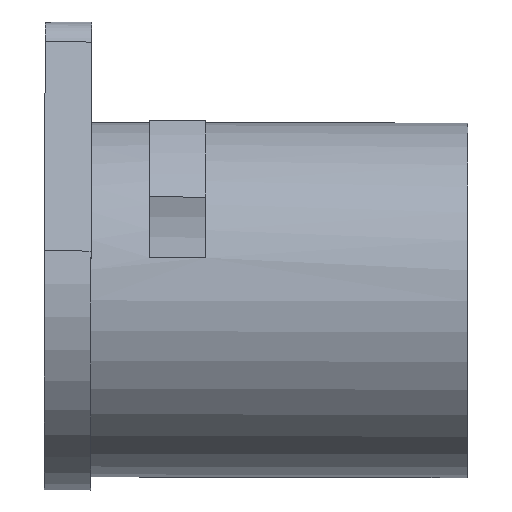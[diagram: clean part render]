
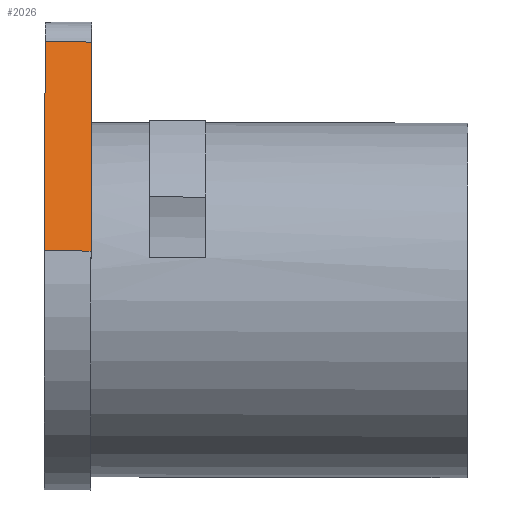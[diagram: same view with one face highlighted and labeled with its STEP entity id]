
A CAD part, left-side view. The second image highlights one B-rep face of the part: STEP entity #2026.
In plain terms, the highlighted planar face has unit normal (-0.967, 0, 0.255).
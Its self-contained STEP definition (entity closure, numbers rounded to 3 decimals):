
#821 = PLANE('',#822);
#822 = AXIS2_PLACEMENT_3D('',#823,#824,#825);
#823 = CARTESIAN_POINT('',(-0.01,-2.316,
    2.141));
#824 = DIRECTION('',(0.,1.,
    0.002));
#825 = DIRECTION('',(1.,0.,
    0.004));
#1085 = VERTEX_POINT('',#1086);
#1086 = CARTESIAN_POINT('',(-9.212,-2.313,
    2.419));
#1105 = CYLINDRICAL_SURFACE('',#1106,9.525);
#1106 = AXIS2_PLACEMENT_3D('',#1107,#1108,#1109);
#1107 = CARTESIAN_POINT('',(0.,0.,0.));
#1108 = DIRECTION('',(0.,-1.,
    -0.002));
#1109 = DIRECTION('',(0.004,0.002,
    -1.));
#1139 = EDGE_CURVE('',#1140,#1085,#1142,.T.);
#1140 = VERTEX_POINT('',#1141);
#1141 = CARTESIAN_POINT('',(-6.469,-2.336,
    12.841));
#1142 = SURFACE_CURVE('',#1143,(#1147,#1154),.PCURVE_S1.);
#1143 = LINE('',#1144,#1145);
#1144 = CARTESIAN_POINT('',(-9.212,-2.313,
    2.419));
#1145 = VECTOR('',#1146,1.);
#1146 = DIRECTION('',(-0.255,0.002,
    -0.967));
#1147 = PCURVE('',#821,#1148);
#1148 = DEFINITIONAL_REPRESENTATION('',(#1149),#1153);
#1149 = LINE('',#1150,#1151);
#1150 = CARTESIAN_POINT('',(-9.2,-0.32));
#1151 = VECTOR('',#1152,1.);
#1152 = DIRECTION('',(-0.259,0.966));
#1153 = ( GEOMETRIC_REPRESENTATION_CONTEXT(2) 
PARAMETRIC_REPRESENTATION_CONTEXT() REPRESENTATION_CONTEXT('2D SPACE',''
  ) );
#1154 = PCURVE('',#1155,#1160);
#1155 = PLANE('',#1156);
#1156 = AXIS2_PLACEMENT_3D('',#1157,#1158,#1159);
#1157 = CARTESIAN_POINT('',(-6.469,-0.025,
    12.846));
#1158 = DIRECTION('',(-0.967,0.,
    0.255));
#1159 = DIRECTION('',(-0.255,0.002,-0.967
    ));
#1160 = DEFINITIONAL_REPRESENTATION('',(#1161),#1165);
#1161 = LINE('',#1162,#1163);
#1162 = CARTESIAN_POINT('',(10.777,2.311));
#1163 = VECTOR('',#1164,1.);
#1164 = DIRECTION('',(1.,0.));
#1165 = ( GEOMETRIC_REPRESENTATION_CONTEXT(2) 
PARAMETRIC_REPRESENTATION_CONTEXT() REPRESENTATION_CONTEXT('2D SPACE',''
  ) );
#1188 = CYLINDRICAL_SURFACE('',#1189,1.27);
#1189 = AXIS2_PLACEMENT_3D('',#1190,#1191,#1192);
#1190 = CARTESIAN_POINT('',(-5.24,-0.024,
    12.523));
#1191 = DIRECTION('',(0.,-1.,
    -0.002));
#1192 = DIRECTION('',(-0.967,0.,
    0.255));
#1531 = PLANE('',#1532);
#1532 = AXIS2_PLACEMENT_3D('',#1533,#1534,#1535);
#1533 = CARTESIAN_POINT('',(-0.01,-0.004,
    2.146));
#1534 = DIRECTION('',(0.,1.,
    0.002));
#1535 = DIRECTION('',(1.,0.,
    0.004));
#1843 = VERTEX_POINT('',#1844);
#1844 = CARTESIAN_POINT('',(-9.211,-0.002,
    2.424));
#1890 = EDGE_CURVE('',#1843,#1085,#1891,.T.);
#1891 = SURFACE_CURVE('',#1892,(#1896,#1925),.PCURVE_S1.);
#1892 = LINE('',#1893,#1894);
#1893 = CARTESIAN_POINT('',(-9.211,-0.002,
    2.424));
#1894 = VECTOR('',#1895,1.);
#1895 = DIRECTION('',(0.,-1.,
    -0.002));
#1896 = PCURVE('',#1105,#1897);
#1897 = DEFINITIONAL_REPRESENTATION('',(#1898),#1924);
#1898 = B_SPLINE_CURVE_WITH_KNOTS('',3,(#1899,#1900,#1901,#1902,#1903,
    #1904,#1905,#1906,#1907,#1908,#1909,#1910,#1911,#1912,#1913,#1914,
    #1915,#1916,#1917,#1918,#1919,#1920,#1921,#1922,#1923),
  .UNSPECIFIED.,.F.,.F.,(4,1,1,1,1,1,1,1,1,1,1,1,1,1,1,1,1,1,1,1,1,1,4),
  (0.,0.105,0.21,0.315,0.42,
    0.525,0.63,0.735,0.841,
    0.946,1.051,1.156,1.261,1.366,
    1.471,1.576,1.681,1.786,
    1.891,1.996,2.101,2.206,2.311),
  .UNSPECIFIED.);
#1899 = CARTESIAN_POINT('',(-1.833,0.));
#1900 = CARTESIAN_POINT('',(-1.833,0.035));
#1901 = CARTESIAN_POINT('',(-1.833,0.105));
#1902 = CARTESIAN_POINT('',(-1.833,0.21));
#1903 = CARTESIAN_POINT('',(-1.833,0.315));
#1904 = CARTESIAN_POINT('',(-1.833,0.42));
#1905 = CARTESIAN_POINT('',(-1.833,0.525));
#1906 = CARTESIAN_POINT('',(-1.833,0.63));
#1907 = CARTESIAN_POINT('',(-1.833,0.735));
#1908 = CARTESIAN_POINT('',(-1.833,0.841));
#1909 = CARTESIAN_POINT('',(-1.833,0.946));
#1910 = CARTESIAN_POINT('',(-1.833,1.051));
#1911 = CARTESIAN_POINT('',(-1.833,1.156));
#1912 = CARTESIAN_POINT('',(-1.833,1.261));
#1913 = CARTESIAN_POINT('',(-1.833,1.366));
#1914 = CARTESIAN_POINT('',(-1.833,1.471));
#1915 = CARTESIAN_POINT('',(-1.833,1.576));
#1916 = CARTESIAN_POINT('',(-1.833,1.681));
#1917 = CARTESIAN_POINT('',(-1.833,1.786));
#1918 = CARTESIAN_POINT('',(-1.833,1.891));
#1919 = CARTESIAN_POINT('',(-1.833,1.996));
#1920 = CARTESIAN_POINT('',(-1.833,2.101));
#1921 = CARTESIAN_POINT('',(-1.833,2.206));
#1922 = CARTESIAN_POINT('',(-1.833,2.276));
#1923 = CARTESIAN_POINT('',(-1.833,2.311));
#1924 = ( GEOMETRIC_REPRESENTATION_CONTEXT(2) 
PARAMETRIC_REPRESENTATION_CONTEXT() REPRESENTATION_CONTEXT('2D SPACE',''
  ) );
#1925 = PCURVE('',#1155,#1926);
#1926 = DEFINITIONAL_REPRESENTATION('',(#1927),#1931);
#1927 = LINE('',#1928,#1929);
#1928 = CARTESIAN_POINT('',(10.777,0.));
#1929 = VECTOR('',#1930,1.);
#1930 = DIRECTION('',(0.,1.));
#1931 = ( GEOMETRIC_REPRESENTATION_CONTEXT(2) 
PARAMETRIC_REPRESENTATION_CONTEXT() REPRESENTATION_CONTEXT('2D SPACE',''
  ) );
#1937 = VERTEX_POINT('',#1938);
#1938 = CARTESIAN_POINT('',(-6.469,-0.025,
    12.846));
#1982 = EDGE_CURVE('',#1937,#1140,#1983,.T.);
#1983 = SURFACE_CURVE('',#1984,(#1988,#2017),.PCURVE_S1.);
#1984 = LINE('',#1985,#1986);
#1985 = CARTESIAN_POINT('',(-6.469,-0.025,
    12.846));
#1986 = VECTOR('',#1987,1.);
#1987 = DIRECTION('',(0.,-1.,
    -0.002));
#1988 = PCURVE('',#1188,#1989);
#1989 = DEFINITIONAL_REPRESENTATION('',(#1990),#2016);
#1990 = B_SPLINE_CURVE_WITH_KNOTS('',3,(#1991,#1992,#1993,#1994,#1995,
    #1996,#1997,#1998,#1999,#2000,#2001,#2002,#2003,#2004,#2005,#2006,
    #2007,#2008,#2009,#2010,#2011,#2012,#2013,#2014,#2015),
  .UNSPECIFIED.,.F.,.F.,(4,1,1,1,1,1,1,1,1,1,1,1,1,1,1,1,1,1,1,1,1,1,4),
  (0.,0.105,0.21,0.315,0.42,
    0.525,0.63,0.735,0.841,
    0.946,1.051,1.156,1.261,1.366,
    1.471,1.576,1.681,1.786,
    1.891,1.996,2.101,2.206,2.311),
  .UNSPECIFIED.);
#1991 = CARTESIAN_POINT('',(6.283,0.));
#1992 = CARTESIAN_POINT('',(6.283,0.035));
#1993 = CARTESIAN_POINT('',(6.283,0.105));
#1994 = CARTESIAN_POINT('',(6.283,0.21));
#1995 = CARTESIAN_POINT('',(6.283,0.315));
#1996 = CARTESIAN_POINT('',(6.283,0.42));
#1997 = CARTESIAN_POINT('',(6.283,0.525));
#1998 = CARTESIAN_POINT('',(6.283,0.63));
#1999 = CARTESIAN_POINT('',(6.283,0.735));
#2000 = CARTESIAN_POINT('',(6.283,0.841));
#2001 = CARTESIAN_POINT('',(6.283,0.946));
#2002 = CARTESIAN_POINT('',(6.283,1.051));
#2003 = CARTESIAN_POINT('',(6.283,1.156));
#2004 = CARTESIAN_POINT('',(6.283,1.261));
#2005 = CARTESIAN_POINT('',(6.283,1.366));
#2006 = CARTESIAN_POINT('',(6.283,1.471));
#2007 = CARTESIAN_POINT('',(6.283,1.576));
#2008 = CARTESIAN_POINT('',(6.283,1.681));
#2009 = CARTESIAN_POINT('',(6.283,1.786));
#2010 = CARTESIAN_POINT('',(6.283,1.891));
#2011 = CARTESIAN_POINT('',(6.283,1.996));
#2012 = CARTESIAN_POINT('',(6.283,2.101));
#2013 = CARTESIAN_POINT('',(6.283,2.206));
#2014 = CARTESIAN_POINT('',(6.283,2.276));
#2015 = CARTESIAN_POINT('',(6.283,2.311));
#2016 = ( GEOMETRIC_REPRESENTATION_CONTEXT(2) 
PARAMETRIC_REPRESENTATION_CONTEXT() REPRESENTATION_CONTEXT('2D SPACE',''
  ) );
#2017 = PCURVE('',#1155,#2018);
#2018 = DEFINITIONAL_REPRESENTATION('',(#2019),#2023);
#2019 = LINE('',#2020,#2021);
#2020 = CARTESIAN_POINT('',(0.,0.));
#2021 = VECTOR('',#2022,1.);
#2022 = DIRECTION('',(0.,1.));
#2023 = ( GEOMETRIC_REPRESENTATION_CONTEXT(2) 
PARAMETRIC_REPRESENTATION_CONTEXT() REPRESENTATION_CONTEXT('2D SPACE',''
  ) );
#2026 = ADVANCED_FACE('',(#2027),#1155,.T.);
#2027 = FACE_BOUND('',#2028,.T.);
#2028 = EDGE_LOOP('',(#2029,#2050,#2051,#2052));
#2029 = ORIENTED_EDGE('',*,*,#2030,.F.);
#2030 = EDGE_CURVE('',#1843,#1937,#2031,.T.);
#2031 = SURFACE_CURVE('',#2032,(#2036,#2043),.PCURVE_S1.);
#2032 = LINE('',#2033,#2034);
#2033 = CARTESIAN_POINT('',(-9.211,-0.002,
    2.424));
#2034 = VECTOR('',#2035,1.);
#2035 = DIRECTION('',(0.255,-0.002,0.967
    ));
#2036 = PCURVE('',#1155,#2037);
#2037 = DEFINITIONAL_REPRESENTATION('',(#2038),#2042);
#2038 = LINE('',#2039,#2040);
#2039 = CARTESIAN_POINT('',(10.777,0.));
#2040 = VECTOR('',#2041,1.);
#2041 = DIRECTION('',(-1.,0.));
#2042 = ( GEOMETRIC_REPRESENTATION_CONTEXT(2) 
PARAMETRIC_REPRESENTATION_CONTEXT() REPRESENTATION_CONTEXT('2D SPACE',''
  ) );
#2043 = PCURVE('',#1531,#2044);
#2044 = DEFINITIONAL_REPRESENTATION('',(#2045),#2049);
#2045 = LINE('',#2046,#2047);
#2046 = CARTESIAN_POINT('',(-9.2,-0.32));
#2047 = VECTOR('',#2048,1.);
#2048 = DIRECTION('',(0.259,-0.966));
#2049 = ( GEOMETRIC_REPRESENTATION_CONTEXT(2) 
PARAMETRIC_REPRESENTATION_CONTEXT() REPRESENTATION_CONTEXT('2D SPACE',''
  ) );
#2050 = ORIENTED_EDGE('',*,*,#1890,.T.);
#2051 = ORIENTED_EDGE('',*,*,#1139,.F.);
#2052 = ORIENTED_EDGE('',*,*,#1982,.F.);
